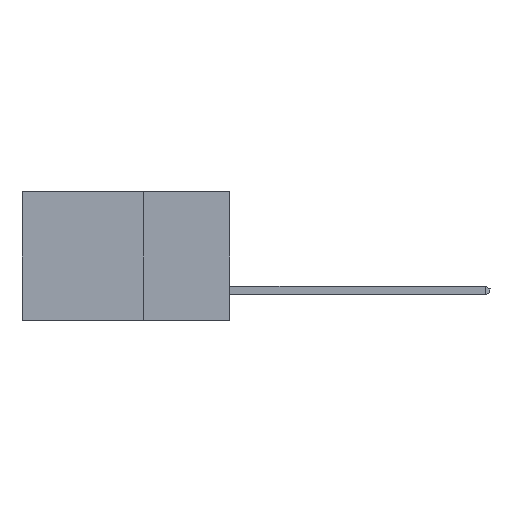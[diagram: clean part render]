
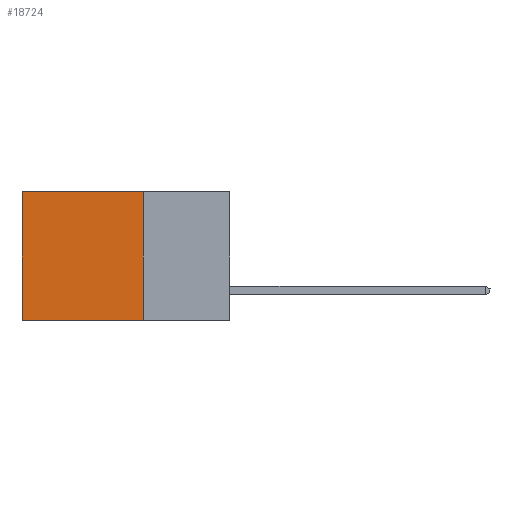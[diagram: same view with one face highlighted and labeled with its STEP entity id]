
A CAD part, left-side view. The second image highlights one B-rep face of the part: STEP entity #18724.
In plain terms, the highlighted planar face has unit normal (-1, 0, 0).
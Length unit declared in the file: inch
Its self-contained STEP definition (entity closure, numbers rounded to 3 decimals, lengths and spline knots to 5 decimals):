
#378 = DIRECTION ( 'NONE',  ( 0., 0., -1. ) ) ;
#721 = LINE ( 'NONE', #7497, #11744 ) ;
#781 = CARTESIAN_POINT ( 'NONE',  ( 0.2615, 0.25, 0. ) ) ;
#1000 = ORIENTED_EDGE ( 'NONE', *, *, #6426, .F. ) ;
#1400 = ORIENTED_EDGE ( 'NONE', *, *, #7304, .F. ) ;
#1609 = PLANE ( 'NONE',  #16743 ) ;
#1658 = VERTEX_POINT ( 'NONE', #18364 ) ;
#3208 = LINE ( 'NONE', #15434, #8895 ) ;
#3423 = ORIENTED_EDGE ( 'NONE', *, *, #7428, .T. ) ;
#3800 = CARTESIAN_POINT ( 'NONE',  ( 0.2615, 0.25, -0.37 ) ) ;
#4103 = CARTESIAN_POINT ( 'NONE',  ( 0.2615, 0.6, 0. ) ) ;
#4564 = DIRECTION ( 'NONE',  ( 0., 1., 0. ) ) ;
#4764 = CARTESIAN_POINT ( 'NONE',  ( 0.2615, 0.25, -0.37 ) ) ;
#5955 = CARTESIAN_POINT ( 'NONE',  ( 0.2615, 0.6, -0.37 ) ) ;
#6315 = VECTOR ( 'NONE', #10708, 39.37008 ) ;
#6426 = EDGE_CURVE ( 'NONE', #7996, #1658, #10489, .T. ) ;
#6573 = DIRECTION ( 'NONE',  ( 0., 0., -1. ) ) ;
#7304 = EDGE_CURVE ( 'NONE', #1658, #15154, #3208, .T. ) ;
#7428 = EDGE_CURVE ( 'NONE', #21966, #15154, #20862, .T. ) ;
#7431 = VECTOR ( 'NONE', #378, 39.37008 ) ;
#7497 = CARTESIAN_POINT ( 'NONE',  ( 0.2615, 0.25, 0. ) ) ;
#7996 = VERTEX_POINT ( 'NONE', #781 ) ;
#8895 = VECTOR ( 'NONE', #4564, 39.37008 ) ;
#10489 = LINE ( 'NONE', #3800, #6315 ) ;
#10708 = DIRECTION ( 'NONE',  ( 0., 0., -1. ) ) ;
#11744 = VECTOR ( 'NONE', #21211, 39.37008 ) ;
#11906 = DIRECTION ( 'NONE',  ( 1., 0., 0. ) ) ;
#12348 = CARTESIAN_POINT ( 'NONE',  ( 0.2615, 0.6, -0.37 ) ) ;
#15154 = VERTEX_POINT ( 'NONE', #5955 ) ;
#15434 = CARTESIAN_POINT ( 'NONE',  ( 0.2615, 0.25, -0.37 ) ) ;
#16743 = AXIS2_PLACEMENT_3D ( 'NONE', #4764, #11906, #6573 ) ;
#17112 = FACE_OUTER_BOUND ( 'NONE', #19116, .T. ) ;
#18364 = CARTESIAN_POINT ( 'NONE',  ( 0.2615, 0.25, -0.37 ) ) ;
#18724 = ADVANCED_FACE ( 'NONE', ( #17112 ), #1609, .F. ) ;
#19116 = EDGE_LOOP ( 'NONE', ( #3423, #1400, #1000, #20454 ) ) ;
#20454 = ORIENTED_EDGE ( 'NONE', *, *, #20646, .T. ) ;
#20646 = EDGE_CURVE ( 'NONE', #7996, #21966, #721, .T. ) ;
#20862 = LINE ( 'NONE', #12348, #7431 ) ;
#21211 = DIRECTION ( 'NONE',  ( 0., 1., 0. ) ) ;
#21966 = VERTEX_POINT ( 'NONE', #4103 ) ;
